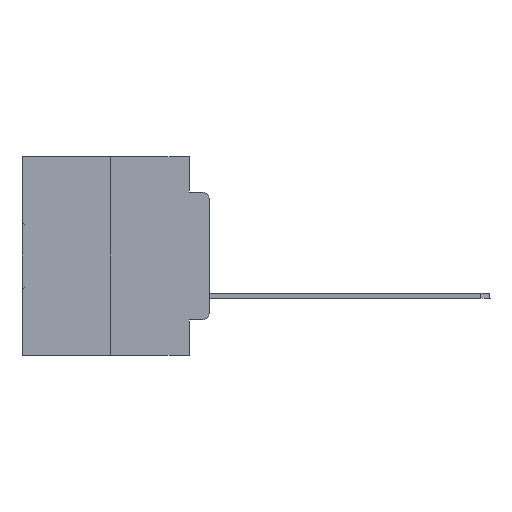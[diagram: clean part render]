
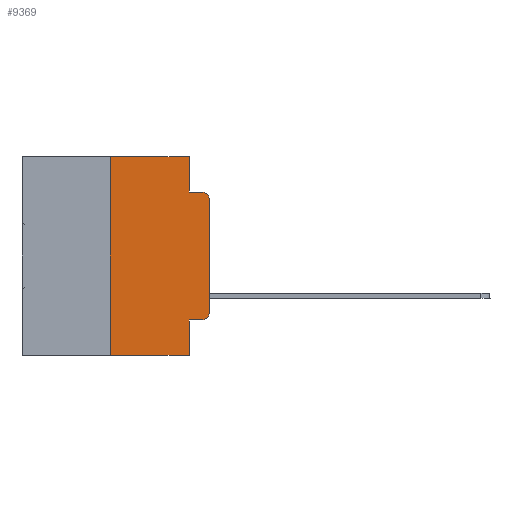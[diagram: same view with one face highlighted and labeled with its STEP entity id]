
A CAD part, left-side view. The second image highlights one B-rep face of the part: STEP entity #9369.
In plain terms, the highlighted planar face has unit normal (-1, 0, 0).
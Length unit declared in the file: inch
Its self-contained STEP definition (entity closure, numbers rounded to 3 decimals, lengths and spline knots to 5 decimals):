
#192 = CARTESIAN_POINT ( 'NONE',  ( 0., 0., -0.3915 ) ) ;
#352 = DIRECTION ( 'NONE',  ( -1., 0., 0. ) ) ;
#723 = DIRECTION ( 'NONE',  ( -1., 0., 0. ) ) ;
#1094 = DIRECTION ( 'NONE',  ( 0., 0., -1. ) ) ;
#1766 = DIRECTION ( 'NONE',  ( 0., 0., -1. ) ) ;
#2554 = DIRECTION ( 'NONE',  ( 0., 0., 1. ) ) ;
#2587 = EDGE_CURVE ( 'NONE', #33303, #29713, #32809, .T. ) ;
#2913 = CARTESIAN_POINT ( 'NONE',  ( 0., 0., -0.1085 ) ) ;
#4036 = CARTESIAN_POINT ( 'NONE',  ( 0., 0.051, 0. ) ) ;
#4450 = VECTOR ( 'NONE', #7002, 39.37008 ) ;
#4549 = EDGE_CURVE ( 'NONE', #15000, #26556, #17284, .T. ) ;
#5771 = CARTESIAN_POINT ( 'NONE',  ( 0., 0.051, -0.0885 ) ) ;
#6017 = CARTESIAN_POINT ( 'NONE',  ( 0., 0.25, 0. ) ) ;
#6781 = VECTOR ( 'NONE', #16472, 39.37008 ) ;
#7002 = DIRECTION ( 'NONE',  ( 0., -1., 0. ) ) ;
#7127 = CARTESIAN_POINT ( 'NONE',  ( 0., 0.473, 0. ) ) ;
#7367 = LINE ( 'NONE', #25541, #11437 ) ;
#7371 = ORIENTED_EDGE ( 'NONE', *, *, #20338, .T. ) ;
#7609 = ORIENTED_EDGE ( 'NONE', *, *, #32133, .F. ) ;
#8385 = LINE ( 'NONE', #28016, #19726 ) ;
#8788 = LINE ( 'NONE', #29098, #6781 ) ;
#9170 = ORIENTED_EDGE ( 'NONE', *, *, #27207, .T. ) ;
#9369 = ADVANCED_FACE ( 'NONE', ( #18568 ), #30524, .F. ) ;
#9854 = DIRECTION ( 'NONE',  ( 0., 0., 1. ) ) ;
#10511 = ORIENTED_EDGE ( 'NONE', *, *, #33301, .T. ) ;
#10879 = VERTEX_POINT ( 'NONE', #11520 ) ;
#11287 = VERTEX_POINT ( 'NONE', #27486 ) ;
#11317 = CARTESIAN_POINT ( 'NONE',  ( 0., 0.02, -0.0885 ) ) ;
#11437 = VECTOR ( 'NONE', #9854, 39.37008 ) ;
#11520 = CARTESIAN_POINT ( 'NONE',  ( 0., 0.25, -0.5 ) ) ;
#12131 = DIRECTION ( 'NONE',  ( 0., 0., -1. ) ) ;
#12746 = EDGE_CURVE ( 'NONE', #10879, #29713, #8788, .T. ) ;
#12875 = ORIENTED_EDGE ( 'NONE', *, *, #25802, .F. ) ;
#13370 = VECTOR ( 'NONE', #1094, 39.37008 ) ;
#14192 = ORIENTED_EDGE ( 'NONE', *, *, #26928, .F. ) ;
#14369 = CARTESIAN_POINT ( 'NONE',  ( 0., 0.051, 0. ) ) ;
#15000 = VERTEX_POINT ( 'NONE', #192 ) ;
#15247 = CARTESIAN_POINT ( 'NONE',  ( 0., 0.051, -0.4115 ) ) ;
#15341 = DIRECTION ( 'NONE',  ( 0., -1., 0. ) ) ;
#15602 = CARTESIAN_POINT ( 'NONE',  ( 0., 0.02, -0.3915 ) ) ;
#16472 = DIRECTION ( 'NONE',  ( 0., -1., 0. ) ) ;
#17284 = LINE ( 'NONE', #23083, #25750 ) ;
#18302 = VECTOR ( 'NONE', #12131, 39.37008 ) ;
#18440 = DIRECTION ( 'NONE',  ( 0., 0., -1. ) ) ;
#18568 = FACE_OUTER_BOUND ( 'NONE', #19407, .T. ) ;
#18882 = CARTESIAN_POINT ( 'NONE',  ( 0., 0.051, -0.5 ) ) ;
#18999 = VECTOR ( 'NONE', #31386, 39.37008 ) ;
#19407 = EDGE_LOOP ( 'NONE', ( #32992, #9170, #7609, #14192, #31906, #12875, #20743, #23119, #10511, #7371 ) ) ;
#19703 = EDGE_CURVE ( 'NONE', #23328, #32488, #29056, .T. ) ;
#19726 = VECTOR ( 'NONE', #15341, 39.37008 ) ;
#19867 = LINE ( 'NONE', #4036, #13370 ) ;
#19869 = CARTESIAN_POINT ( 'NONE',  ( 0., 0.051, 0. ) ) ;
#20016 = CARTESIAN_POINT ( 'NONE',  ( 0., 0.473, 0. ) ) ;
#20338 = EDGE_CURVE ( 'NONE', #11287, #15000, #25406, .T. ) ;
#20509 = AXIS2_PLACEMENT_3D ( 'NONE', #7127, #25451, #1766 ) ;
#20743 = ORIENTED_EDGE ( 'NONE', *, *, #12746, .T. ) ;
#22441 = VERTEX_POINT ( 'NONE', #30556 ) ;
#22872 = CARTESIAN_POINT ( 'NONE',  ( 0., 0.02, -0.1085 ) ) ;
#23083 = CARTESIAN_POINT ( 'NONE',  ( 0., 0., 0. ) ) ;
#23119 = ORIENTED_EDGE ( 'NONE', *, *, #2587, .F. ) ;
#23328 = VERTEX_POINT ( 'NONE', #6017 ) ;
#25406 = CIRCLE ( 'NONE', #29158, 0.02 ) ;
#25451 = DIRECTION ( 'NONE',  ( 1., 0., 0. ) ) ;
#25504 = LINE ( 'NONE', #5771, #18999 ) ;
#25541 = CARTESIAN_POINT ( 'NONE',  ( 0., 0.25, 0. ) ) ;
#25750 = VECTOR ( 'NONE', #2554, 39.37008 ) ;
#25802 = EDGE_CURVE ( 'NONE', #10879, #23328, #7367, .T. ) ;
#26288 = CIRCLE ( 'NONE', #29106, 0.02 ) ;
#26556 = VERTEX_POINT ( 'NONE', #2913 ) ;
#26928 = EDGE_CURVE ( 'NONE', #32488, #22441, #19867, .T. ) ;
#27207 = EDGE_CURVE ( 'NONE', #26556, #29699, #26288, .T. ) ;
#27486 = CARTESIAN_POINT ( 'NONE',  ( 0., 0.02, -0.4115 ) ) ;
#28016 = CARTESIAN_POINT ( 'NONE',  ( 0., 0.051, -0.4115 ) ) ;
#29056 = LINE ( 'NONE', #20016, #4450 ) ;
#29098 = CARTESIAN_POINT ( 'NONE',  ( 0., 0.473, -0.5 ) ) ;
#29106 = AXIS2_PLACEMENT_3D ( 'NONE', #22872, #723, #31479 ) ;
#29158 = AXIS2_PLACEMENT_3D ( 'NONE', #15602, #352, #18440 ) ;
#29699 = VERTEX_POINT ( 'NONE', #11317 ) ;
#29713 = VERTEX_POINT ( 'NONE', #18882 ) ;
#30524 = PLANE ( 'NONE',  #20509 ) ;
#30556 = CARTESIAN_POINT ( 'NONE',  ( 0., 0.051, -0.0885 ) ) ;
#31386 = DIRECTION ( 'NONE',  ( 0., -1., 0. ) ) ;
#31479 = DIRECTION ( 'NONE',  ( 0., 0., -1. ) ) ;
#31906 = ORIENTED_EDGE ( 'NONE', *, *, #19703, .F. ) ;
#32133 = EDGE_CURVE ( 'NONE', #22441, #29699, #25504, .T. ) ;
#32488 = VERTEX_POINT ( 'NONE', #14369 ) ;
#32809 = LINE ( 'NONE', #19869, #18302 ) ;
#32992 = ORIENTED_EDGE ( 'NONE', *, *, #4549, .T. ) ;
#33301 = EDGE_CURVE ( 'NONE', #33303, #11287, #8385, .T. ) ;
#33303 = VERTEX_POINT ( 'NONE', #15247 ) ;
